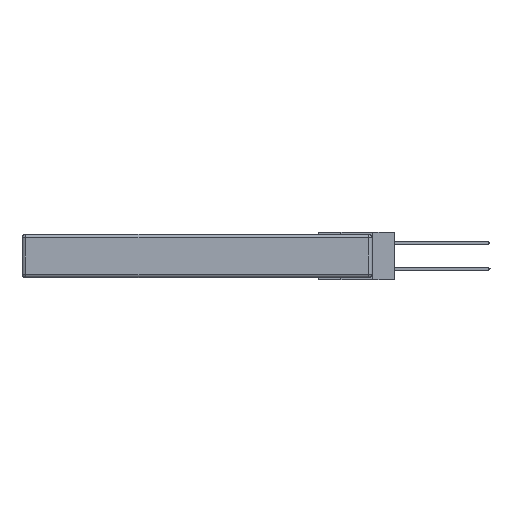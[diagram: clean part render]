
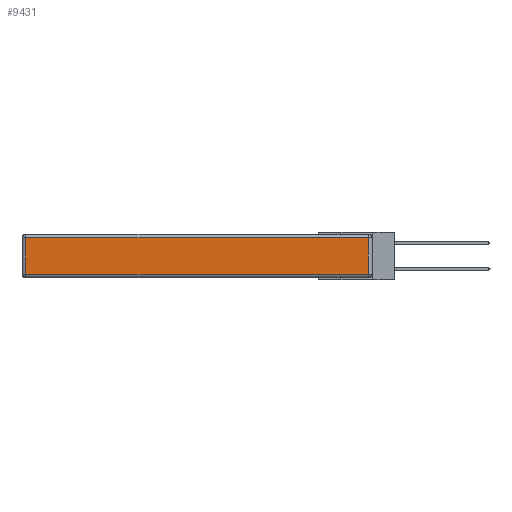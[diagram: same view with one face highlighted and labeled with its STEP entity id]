
A CAD part, left-side view. The second image highlights one B-rep face of the part: STEP entity #9431.
In plain terms, the highlighted planar face has unit normal (-1, 0, 0).
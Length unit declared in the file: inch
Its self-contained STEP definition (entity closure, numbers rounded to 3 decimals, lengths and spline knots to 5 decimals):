
#140 = EDGE_CURVE ( 'NONE', #7771, #10081, #9858, .T. ) ;
#468 = CARTESIAN_POINT ( 'NONE',  ( 0., 2.72, -0.313 ) ) ;
#1496 = CARTESIAN_POINT ( 'NONE',  ( 0., 0.03, -0.03 ) ) ;
#1620 = EDGE_LOOP ( 'NONE', ( #6914, #5815, #12192, #17778 ) ) ;
#1770 = CARTESIAN_POINT ( 'NONE',  ( 0., 2.72, -0.343 ) ) ;
#2769 = CARTESIAN_POINT ( 'NONE',  ( 0., 0.03, -0.343 ) ) ;
#2903 = DIRECTION ( 'NONE',  ( -1., 0., 0. ) ) ;
#3605 = EDGE_CURVE ( 'NONE', #10081, #19163, #22531, .T. ) ;
#4685 = CARTESIAN_POINT ( 'NONE',  ( 0., 0., -0.343 ) ) ;
#5815 = ORIENTED_EDGE ( 'NONE', *, *, #9118, .T. ) ;
#6451 = DIRECTION ( 'NONE',  ( 0., 1., 0. ) ) ;
#6914 = ORIENTED_EDGE ( 'NONE', *, *, #3605, .T. ) ;
#7363 = CARTESIAN_POINT ( 'NONE',  ( 0., 0., -0.313 ) ) ;
#7738 = CARTESIAN_POINT ( 'NONE',  ( 0., 0.03, -0.313 ) ) ;
#7771 = VERTEX_POINT ( 'NONE', #15369 ) ;
#8263 = DIRECTION ( 'NONE',  ( 0., 0., 1. ) ) ;
#8463 = VECTOR ( 'NONE', #17348, 39.37008 ) ;
#9118 = EDGE_CURVE ( 'NONE', #19163, #21583, #10766, .T. ) ;
#9431 = ADVANCED_FACE ( 'NONE', ( #18156 ), #21166, .T. ) ;
#9858 = LINE ( 'NONE', #1770, #11586 ) ;
#10081 = VERTEX_POINT ( 'NONE', #468 ) ;
#10766 = LINE ( 'NONE', #2769, #8463 ) ;
#11586 = VECTOR ( 'NONE', #22126, 39.37008 ) ;
#12192 = ORIENTED_EDGE ( 'NONE', *, *, #20356, .T. ) ;
#13600 = CARTESIAN_POINT ( 'NONE',  ( 0., 2.75, -0.03 ) ) ;
#15369 = CARTESIAN_POINT ( 'NONE',  ( 0., 2.72, -0.03 ) ) ;
#17348 = DIRECTION ( 'NONE',  ( 0., 0., 1. ) ) ;
#17560 = VECTOR ( 'NONE', #6451, 39.37008 ) ;
#17644 = VECTOR ( 'NONE', #18594, 39.37008 ) ;
#17778 = ORIENTED_EDGE ( 'NONE', *, *, #140, .T. ) ;
#18156 = FACE_OUTER_BOUND ( 'NONE', #1620, .T. ) ;
#18594 = DIRECTION ( 'NONE',  ( 0., -1., 0. ) ) ;
#19163 = VERTEX_POINT ( 'NONE', #7738 ) ;
#20356 = EDGE_CURVE ( 'NONE', #21583, #7771, #22448, .T. ) ;
#20379 = AXIS2_PLACEMENT_3D ( 'NONE', #4685, #2903, #8263 ) ;
#21166 = PLANE ( 'NONE',  #20379 ) ;
#21583 = VERTEX_POINT ( 'NONE', #1496 ) ;
#22126 = DIRECTION ( 'NONE',  ( 0., 0., -1. ) ) ;
#22448 = LINE ( 'NONE', #13600, #17560 ) ;
#22531 = LINE ( 'NONE', #7363, #17644 ) ;
